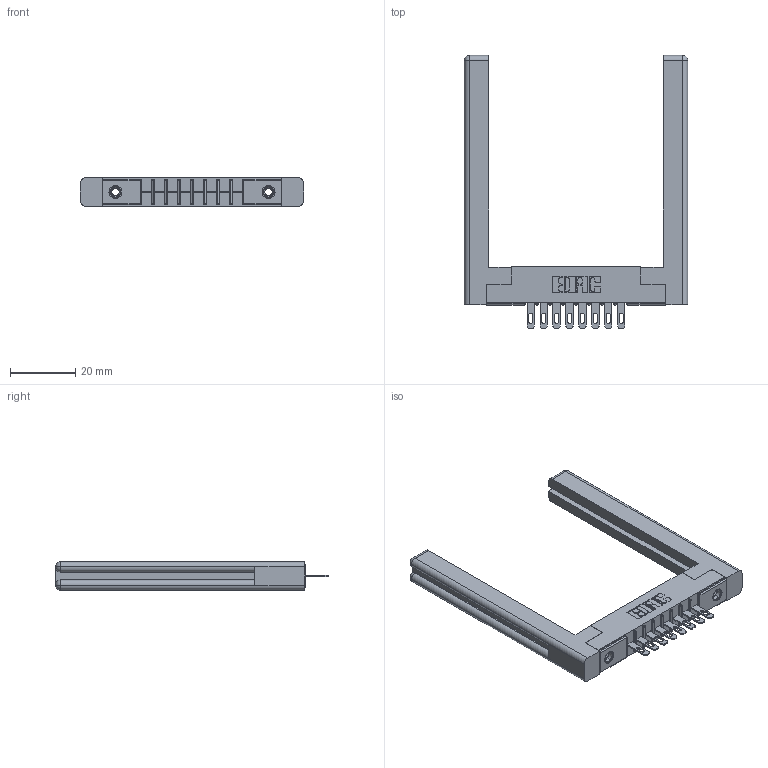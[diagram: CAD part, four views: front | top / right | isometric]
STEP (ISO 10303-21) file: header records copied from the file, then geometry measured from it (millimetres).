
FILE_DESCRIPTION (( 'STEP AP203' ), '1' );
FILE_NAME ('316-008-400-158.STEP', '2020-09-22T14:28:43', ( '' ), ( '' ), 'SwSTEP 2.0', 'SolidWorks 2020', '' );
FILE_SCHEMA (( 'CONFIG_CONTROL_DESIGN' ));
Length unit declared in the file: inch
Products named in the file (5): 306 Part_.156 Dia; 307-220-058; 345-250-001_345-250-001-102; 316-008-400-158; 306-290-001_100
Assembly tree (13 placements, depth 2):
  316-008-400-158
    306 Part_.156 Dia
    306-290-001_100  x8
    345-250-001_345-250-001-102  x2
    307-220-058  x2
Bounding box: 68.33 x 83.52 x 8.71 mm (x, y, z)
Volume: 12286.9 mm3; surface area: 11829.2 mm2
Topology: 13 solids, 13 shells, 866 faces, 2390 edges, 1536 vertices
Faces by surface type: plane 552, cylinder 258, sphere 32, cone 12, torus 12
Entity records: 14662 total; most frequent: CARTESIAN_POINT 2466, DIRECTION 2391, ORIENTED_EDGE 2382, EDGE_CURVE 1191, LINE 905, VECTOR 905, VERTEX_POINT 764, AXIS2_PLACEMENT_3D 743
